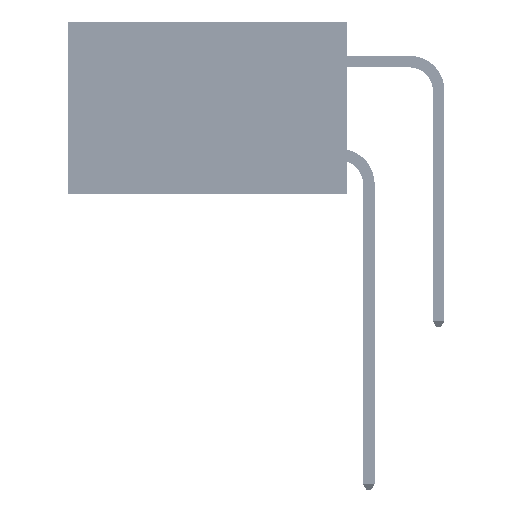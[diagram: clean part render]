
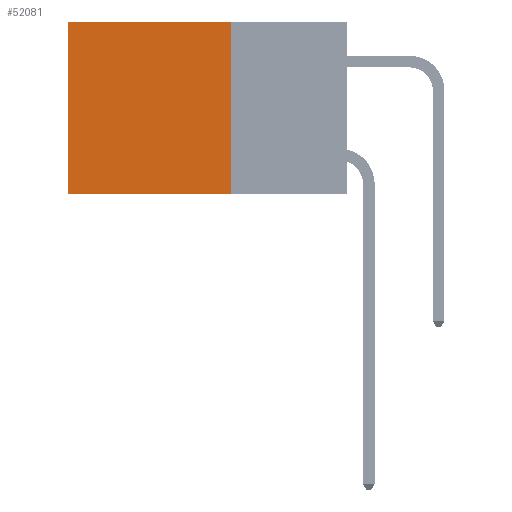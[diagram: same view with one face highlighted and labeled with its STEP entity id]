
A CAD part, left-side view. The second image highlights one B-rep face of the part: STEP entity #52081.
In plain terms, the highlighted planar face has unit normal (-1, 0, 0).
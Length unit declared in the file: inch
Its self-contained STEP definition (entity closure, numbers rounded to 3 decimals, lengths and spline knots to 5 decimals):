
#2385 = FACE_OUTER_BOUND ( 'NONE', #35735, .T. ) ;
#3125 = EDGE_CURVE ( 'NONE', #12922, #24045, #32940, .T. ) ;
#6005 = CARTESIAN_POINT ( 'NONE',  ( 0.2875, 0.6, 0. ) ) ;
#8053 = CARTESIAN_POINT ( 'NONE',  ( 0.2875, 0.6, -0.37 ) ) ;
#10000 = AXIS2_PLACEMENT_3D ( 'NONE', #19910, #44747, #44576 ) ;
#11640 = PLANE ( 'NONE',  #10000 ) ;
#12118 = ORIENTED_EDGE ( 'NONE', *, *, #3125, .T. ) ;
#12922 = VERTEX_POINT ( 'NONE', #6005 ) ;
#12980 = ORIENTED_EDGE ( 'NONE', *, *, #45686, .F. ) ;
#13907 = DIRECTION ( 'NONE',  ( 0., 0., -1. ) ) ;
#14028 = VECTOR ( 'NONE', #13907, 39.37008 ) ;
#14192 = EDGE_CURVE ( 'NONE', #50908, #24045, #48486, .T. ) ;
#17285 = ORIENTED_EDGE ( 'NONE', *, *, #34965, .T. ) ;
#17619 = VECTOR ( 'NONE', #30926, 39.37008 ) ;
#18420 = LINE ( 'NONE', #40016, #49313 ) ;
#19399 = DIRECTION ( 'NONE',  ( 0., 1., 0. ) ) ;
#19910 = CARTESIAN_POINT ( 'NONE',  ( 0.2875, 0.25, 0. ) ) ;
#24045 = VERTEX_POINT ( 'NONE', #8053 ) ;
#24099 = VERTEX_POINT ( 'NONE', #45060 ) ;
#30926 = DIRECTION ( 'NONE',  ( 0., 1., 0. ) ) ;
#32940 = LINE ( 'NONE', #37841, #14028 ) ;
#34778 = DIRECTION ( 'NONE',  ( 0., 0., -1. ) ) ;
#34965 = EDGE_CURVE ( 'NONE', #24099, #12922, #18420, .T. ) ;
#35735 = EDGE_LOOP ( 'NONE', ( #12118, #48779, #12980, #17285 ) ) ;
#35853 = VECTOR ( 'NONE', #34778, 39.37008 ) ;
#37838 = CARTESIAN_POINT ( 'NONE',  ( 0.2875, 0.25, -0.37 ) ) ;
#37841 = CARTESIAN_POINT ( 'NONE',  ( 0.2875, 0.6, 0. ) ) ;
#40016 = CARTESIAN_POINT ( 'NONE',  ( 0.2875, 0.25, 0. ) ) ;
#44576 = DIRECTION ( 'NONE',  ( 0., 0., -1. ) ) ;
#44747 = DIRECTION ( 'NONE',  ( 1., 0., 0. ) ) ;
#45060 = CARTESIAN_POINT ( 'NONE',  ( 0.2875, 0.25, 0. ) ) ;
#45686 = EDGE_CURVE ( 'NONE', #24099, #50908, #47814, .T. ) ;
#46702 = CARTESIAN_POINT ( 'NONE',  ( 0.2875, 0.25, 0. ) ) ;
#47814 = LINE ( 'NONE', #46702, #35853 ) ;
#48486 = LINE ( 'NONE', #50806, #17619 ) ;
#48779 = ORIENTED_EDGE ( 'NONE', *, *, #14192, .F. ) ;
#49313 = VECTOR ( 'NONE', #19399, 39.37008 ) ;
#50806 = CARTESIAN_POINT ( 'NONE',  ( 0.2875, 0.25, -0.37 ) ) ;
#50908 = VERTEX_POINT ( 'NONE', #37838 ) ;
#52081 = ADVANCED_FACE ( 'NONE', ( #2385 ), #11640, .F. ) ;
